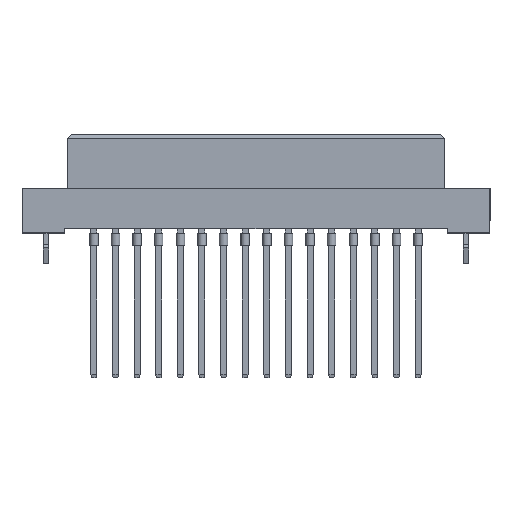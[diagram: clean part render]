
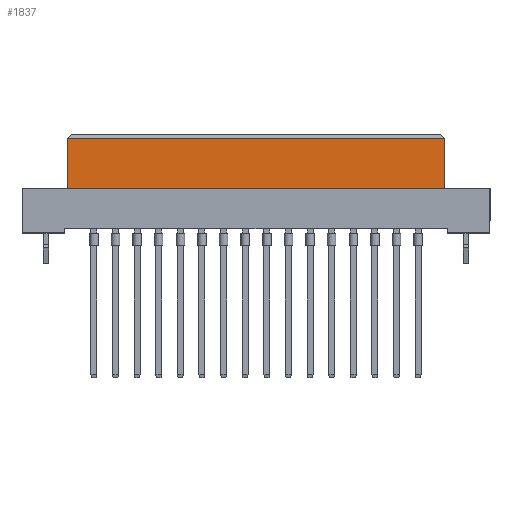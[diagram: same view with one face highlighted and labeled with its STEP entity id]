
A CAD part, top view. The second image highlights one B-rep face of the part: STEP entity #1837.
In plain terms, the highlighted planar face has unit normal (0, 0, 1).
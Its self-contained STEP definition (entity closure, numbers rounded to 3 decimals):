
#1310 = LINE ( 'NONE', #19213, #9270 ) ;
#1837 = ADVANCED_FACE ( 'NONE', ( #21025 ), #15997, .T. ) ;
#1880 = ORIENTED_EDGE ( 'NONE', *, *, #13780, .T. ) ;
#2132 = DIRECTION ( 'NONE',  ( 0., 1., 0. ) ) ;
#2164 = VECTOR ( 'NONE', #5600, 1000. ) ;
#3442 = VERTEX_POINT ( 'NONE', #12965 ) ;
#4827 = DIRECTION ( 'NONE',  ( 0., 0., 1. ) ) ;
#5600 = DIRECTION ( 'NONE',  ( -1., 0., 0. ) ) ;
#6935 = VERTEX_POINT ( 'NONE', #15773 ) ;
#8078 = ORIENTED_EDGE ( 'NONE', *, *, #10180, .T. ) ;
#8444 = CARTESIAN_POINT ( 'NONE',  ( 22.2, -6.4, 4.25 ) ) ;
#9270 = VECTOR ( 'NONE', #11084, 1000. ) ;
#10180 = EDGE_CURVE ( 'NONE', #11179, #3442, #20024, .T. ) ;
#11084 = DIRECTION ( 'NONE',  ( 0., 1., 0. ) ) ;
#11179 = VERTEX_POINT ( 'NONE', #17505 ) ;
#12361 = VECTOR ( 'NONE', #14489, 1000. ) ;
#12743 = VERTEX_POINT ( 'NONE', #19062 ) ;
#12791 = ORIENTED_EDGE ( 'NONE', *, *, #21094, .F. ) ;
#12965 = CARTESIAN_POINT ( 'NONE',  ( 22.2, -0.5, 4.25 ) ) ;
#13190 = VECTOR ( 'NONE', #2132, 1000. ) ;
#13780 = EDGE_CURVE ( 'NONE', #6935, #11179, #19297, .T. ) ;
#14094 = EDGE_LOOP ( 'NONE', ( #8078, #14501, #12791, #1880 ) ) ;
#14386 = CARTESIAN_POINT ( 'NONE',  ( 22.2, -6.4, 4.25 ) ) ;
#14489 = DIRECTION ( 'NONE',  ( 1., 0., 0. ) ) ;
#14501 = ORIENTED_EDGE ( 'NONE', *, *, #16616, .T. ) ;
#15360 = LINE ( 'NONE', #20060, #2164 ) ;
#15773 = CARTESIAN_POINT ( 'NONE',  ( -22.2, -6.4, 4.25 ) ) ;
#15997 = PLANE ( 'NONE',  #16303 ) ;
#16303 = AXIS2_PLACEMENT_3D ( 'NONE', #16410, #4827, #17713 ) ;
#16410 = CARTESIAN_POINT ( 'NONE',  ( 22.2, -6.4, 4.25 ) ) ;
#16616 = EDGE_CURVE ( 'NONE', #3442, #12743, #15360, .T. ) ;
#17505 = CARTESIAN_POINT ( 'NONE',  ( 22.2, -6.4, 4.25 ) ) ;
#17713 = DIRECTION ( 'NONE',  ( 1., 0., 0. ) ) ;
#19062 = CARTESIAN_POINT ( 'NONE',  ( -22.2, -0.5, 4.25 ) ) ;
#19213 = CARTESIAN_POINT ( 'NONE',  ( -22.2, -6.4, 4.25 ) ) ;
#19297 = LINE ( 'NONE', #14386, #12361 ) ;
#20024 = LINE ( 'NONE', #8444, #13190 ) ;
#20060 = CARTESIAN_POINT ( 'NONE',  ( -22.2, -0.5, 4.25 ) ) ;
#21025 = FACE_OUTER_BOUND ( 'NONE', #14094, .T. ) ;
#21094 = EDGE_CURVE ( 'NONE', #6935, #12743, #1310, .T. ) ;
